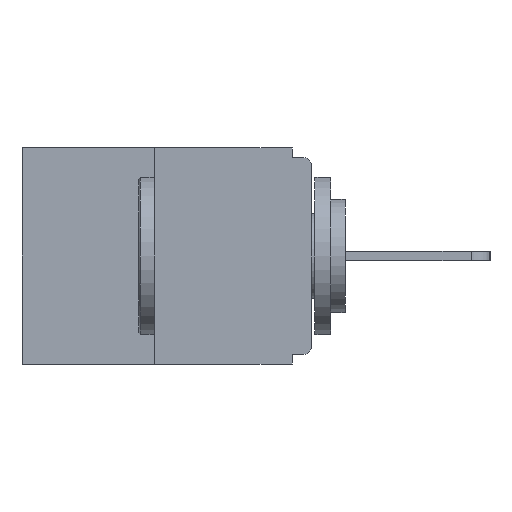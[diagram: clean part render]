
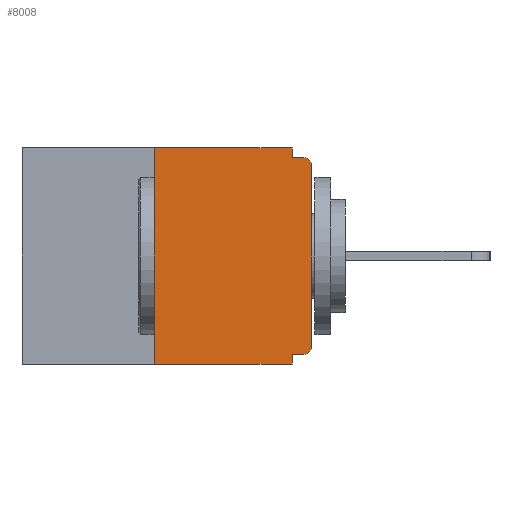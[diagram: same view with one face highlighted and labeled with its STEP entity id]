
A CAD part, left-side view. The second image highlights one B-rep face of the part: STEP entity #8008.
In plain terms, the highlighted planar face has unit normal (-1, 0, 0).
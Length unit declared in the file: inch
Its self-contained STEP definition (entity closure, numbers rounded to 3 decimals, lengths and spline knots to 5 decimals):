
#40 = LINE ( 'NONE', #1765, #6701 ) ;
#305 = VERTEX_POINT ( 'NONE', #6324 ) ;
#585 = DIRECTION ( 'NONE',  ( -1., 0., 0. ) ) ;
#900 = DIRECTION ( 'NONE',  ( 0., -1., 0. ) ) ;
#953 = DIRECTION ( 'NONE',  ( 0., -1., 0. ) ) ;
#1145 = CARTESIAN_POINT ( 'NONE',  ( 0., 0.031, -0.015 ) ) ;
#1185 = VERTEX_POINT ( 'NONE', #1689 ) ;
#1467 = EDGE_CURVE ( 'NONE', #2433, #8027, #5104, .T. ) ;
#1689 = CARTESIAN_POINT ( 'NONE',  ( 0., 0., -0.03 ) ) ;
#1765 = CARTESIAN_POINT ( 'NONE',  ( 0., 0., -0.328 ) ) ;
#1869 = VERTEX_POINT ( 'NONE', #8171 ) ;
#2138 = DIRECTION ( 'NONE',  ( 0., 0., -1. ) ) ;
#2433 = VERTEX_POINT ( 'NONE', #2558 ) ;
#2558 = CARTESIAN_POINT ( 'NONE',  ( 0., 0.015, -0.328 ) ) ;
#2714 = ORIENTED_EDGE ( 'NONE', *, *, #5648, .F. ) ;
#3215 = PLANE ( 'NONE',  #13540 ) ;
#3594 = CARTESIAN_POINT ( 'NONE',  ( 0., 0.031, -0.343 ) ) ;
#3922 = ORIENTED_EDGE ( 'NONE', *, *, #18875, .F. ) ;
#4171 = EDGE_CURVE ( 'NONE', #11342, #305, #12583, .T. ) ;
#4516 = VERTEX_POINT ( 'NONE', #16924 ) ;
#4871 = VERTEX_POINT ( 'NONE', #10384 ) ;
#5104 = CIRCLE ( 'NONE', #10967, 0.015 ) ;
#5648 = EDGE_CURVE ( 'NONE', #4516, #305, #18477, .T. ) ;
#6166 = CARTESIAN_POINT ( 'NONE',  ( 0., 0.46, -0.343 ) ) ;
#6324 = CARTESIAN_POINT ( 'NONE',  ( 0., 0.031, -0.343 ) ) ;
#6571 = EDGE_CURVE ( 'NONE', #1185, #1869, #8175, .T. ) ;
#6701 = VECTOR ( 'NONE', #16175, 39.37008 ) ;
#6953 = CARTESIAN_POINT ( 'NONE',  ( 0., 0.25, 0. ) ) ;
#6982 = EDGE_CURVE ( 'NONE', #11342, #17159, #20011, .T. ) ;
#7339 = CARTESIAN_POINT ( 'NONE',  ( 0., 0.031, 0. ) ) ;
#7512 = VERTEX_POINT ( 'NONE', #1145 ) ;
#7932 = CARTESIAN_POINT ( 'NONE',  ( 0., 0.46, 0. ) ) ;
#8008 = ADVANCED_FACE ( 'NONE', ( #12649 ), #3215, .F. ) ;
#8027 = VERTEX_POINT ( 'NONE', #19074 ) ;
#8171 = CARTESIAN_POINT ( 'NONE',  ( 0., 0.015, -0.015 ) ) ;
#8175 = CIRCLE ( 'NONE', #9199, 0.015 ) ;
#8349 = CARTESIAN_POINT ( 'NONE',  ( 0., 0.25, -0.343 ) ) ;
#9015 = LINE ( 'NONE', #15537, #14925 ) ;
#9016 = CARTESIAN_POINT ( 'NONE',  ( 0., 0.015, -0.03 ) ) ;
#9199 = AXIS2_PLACEMENT_3D ( 'NONE', #9016, #585, #20151 ) ;
#9801 = EDGE_CURVE ( 'NONE', #2433, #4516, #40, .T. ) ;
#10082 = VECTOR ( 'NONE', #953, 39.37008 ) ;
#10309 = DIRECTION ( 'NONE',  ( 0., -1., 0. ) ) ;
#10384 = CARTESIAN_POINT ( 'NONE',  ( 0., 0.031, 0. ) ) ;
#10967 = AXIS2_PLACEMENT_3D ( 'NONE', #13531, #11385, #17905 ) ;
#11315 = ORIENTED_EDGE ( 'NONE', *, *, #1467, .T. ) ;
#11342 = VERTEX_POINT ( 'NONE', #8349 ) ;
#11385 = DIRECTION ( 'NONE',  ( -1., 0., 0. ) ) ;
#11795 = VECTOR ( 'NONE', #12136, 39.37008 ) ;
#12136 = DIRECTION ( 'NONE',  ( 0., 0., -1. ) ) ;
#12295 = EDGE_LOOP ( 'NONE', ( #12860, #12931, #20103, #2714, #13723, #11315, #13325, #12494, #3922, #13615 ) ) ;
#12494 = ORIENTED_EDGE ( 'NONE', *, *, #6571, .T. ) ;
#12583 = LINE ( 'NONE', #6166, #10082 ) ;
#12649 = FACE_OUTER_BOUND ( 'NONE', #12295, .T. ) ;
#12860 = ORIENTED_EDGE ( 'NONE', *, *, #19913, .F. ) ;
#12878 = LINE ( 'NONE', #14091, #15578 ) ;
#12931 = ORIENTED_EDGE ( 'NONE', *, *, #6982, .F. ) ;
#13325 = ORIENTED_EDGE ( 'NONE', *, *, #16529, .T. ) ;
#13397 = CARTESIAN_POINT ( 'NONE',  ( 0., 0.25, 0. ) ) ;
#13531 = CARTESIAN_POINT ( 'NONE',  ( 0., 0.015, -0.313 ) ) ;
#13540 = AXIS2_PLACEMENT_3D ( 'NONE', #7932, #14469, #19179 ) ;
#13615 = ORIENTED_EDGE ( 'NONE', *, *, #16346, .F. ) ;
#13633 = CARTESIAN_POINT ( 'NONE',  ( 0., 0.46, 0. ) ) ;
#13723 = ORIENTED_EDGE ( 'NONE', *, *, #9801, .F. ) ;
#14091 = CARTESIAN_POINT ( 'NONE',  ( 0., 0., 0. ) ) ;
#14469 = DIRECTION ( 'NONE',  ( 1., 0., 0. ) ) ;
#14925 = VECTOR ( 'NONE', #900, 39.37008 ) ;
#15310 = VECTOR ( 'NONE', #10309, 39.37008 ) ;
#15537 = CARTESIAN_POINT ( 'NONE',  ( 0., 0., -0.015 ) ) ;
#15578 = VECTOR ( 'NONE', #17388, 39.37008 ) ;
#16175 = DIRECTION ( 'NONE',  ( 0., 1., 0. ) ) ;
#16346 = EDGE_CURVE ( 'NONE', #4871, #7512, #17176, .T. ) ;
#16529 = EDGE_CURVE ( 'NONE', #8027, #1185, #12878, .T. ) ;
#16924 = CARTESIAN_POINT ( 'NONE',  ( 0., 0.031, -0.328 ) ) ;
#17159 = VERTEX_POINT ( 'NONE', #13397 ) ;
#17176 = LINE ( 'NONE', #7339, #11795 ) ;
#17388 = DIRECTION ( 'NONE',  ( 0., 0., 1. ) ) ;
#17738 = VECTOR ( 'NONE', #18721, 39.37008 ) ;
#17905 = DIRECTION ( 'NONE',  ( 0., 0., -1. ) ) ;
#18319 = LINE ( 'NONE', #13633, #15310 ) ;
#18477 = LINE ( 'NONE', #3594, #21042 ) ;
#18721 = DIRECTION ( 'NONE',  ( 0., 0., 1. ) ) ;
#18875 = EDGE_CURVE ( 'NONE', #7512, #1869, #9015, .T. ) ;
#19074 = CARTESIAN_POINT ( 'NONE',  ( 0., 0., -0.313 ) ) ;
#19179 = DIRECTION ( 'NONE',  ( 0., 0., -1. ) ) ;
#19913 = EDGE_CURVE ( 'NONE', #17159, #4871, #18319, .T. ) ;
#20011 = LINE ( 'NONE', #6953, #17738 ) ;
#20103 = ORIENTED_EDGE ( 'NONE', *, *, #4171, .T. ) ;
#20151 = DIRECTION ( 'NONE',  ( 0., 0., -1. ) ) ;
#21042 = VECTOR ( 'NONE', #2138, 39.37008 ) ;
